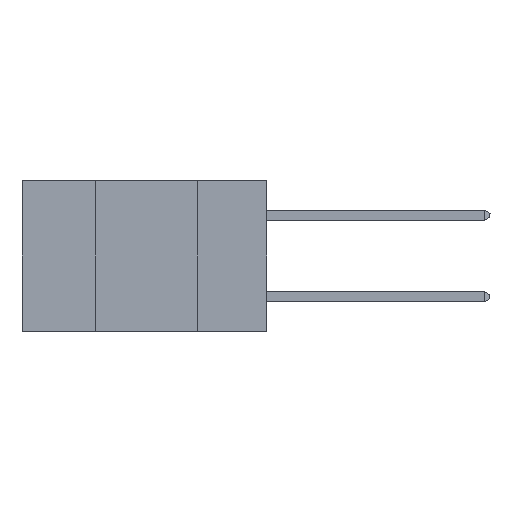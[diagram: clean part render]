
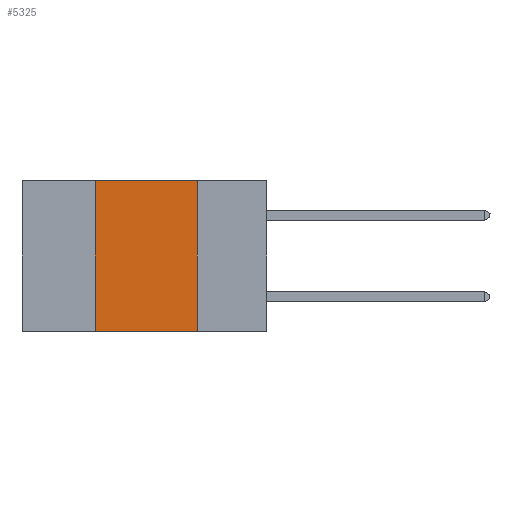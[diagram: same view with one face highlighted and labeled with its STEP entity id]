
A CAD part, left-side view. The second image highlights one B-rep face of the part: STEP entity #5325.
In plain terms, the highlighted planar face has unit normal (-1, 0, 0).
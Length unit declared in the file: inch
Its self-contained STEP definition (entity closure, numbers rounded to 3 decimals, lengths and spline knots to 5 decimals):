
#87 = DIRECTION ( 'NONE',  ( 0., -1., 0. ) ) ;
#696 = ORIENTED_EDGE ( 'NONE', *, *, #19331, .F. ) ;
#1381 = ORIENTED_EDGE ( 'NONE', *, *, #11304, .F. ) ;
#1955 = CARTESIAN_POINT ( 'NONE',  ( 0., 0.6, 0. ) ) ;
#4219 = CARTESIAN_POINT ( 'NONE',  ( 0., 0.17, -0.37 ) ) ;
#5291 = CARTESIAN_POINT ( 'NONE',  ( 0., 0.42, 0. ) ) ;
#5325 = ADVANCED_FACE ( 'NONE', ( #12590 ), #6819, .F. ) ;
#5712 = LINE ( 'NONE', #8011, #13206 ) ;
#6655 = DIRECTION ( 'NONE',  ( 0., 0., -1. ) ) ;
#6819 = PLANE ( 'NONE',  #17842 ) ;
#7284 = VERTEX_POINT ( 'NONE', #9125 ) ;
#7323 = DIRECTION ( 'NONE',  ( 1., 0., 0. ) ) ;
#7346 = VECTOR ( 'NONE', #11225, 39.37008 ) ;
#8011 = CARTESIAN_POINT ( 'NONE',  ( 0., 0.6, -0.37 ) ) ;
#8307 = DIRECTION ( 'NONE',  ( 0., 0., 1. ) ) ;
#8424 = ORIENTED_EDGE ( 'NONE', *, *, #16212, .F. ) ;
#8816 = VERTEX_POINT ( 'NONE', #12706 ) ;
#9031 = ORIENTED_EDGE ( 'NONE', *, *, #18347, .T. ) ;
#9125 = CARTESIAN_POINT ( 'NONE',  ( 0., 0.42, 0. ) ) ;
#10148 = DIRECTION ( 'NONE',  ( 0., 0., -1. ) ) ;
#10223 = VERTEX_POINT ( 'NONE', #4219 ) ;
#11225 = DIRECTION ( 'NONE',  ( 0., -1., 0. ) ) ;
#11304 = EDGE_CURVE ( 'NONE', #15109, #7284, #18231, .T. ) ;
#11358 = VECTOR ( 'NONE', #10148, 39.37008 ) ;
#12590 = FACE_OUTER_BOUND ( 'NONE', #13124, .T. ) ;
#12706 = CARTESIAN_POINT ( 'NONE',  ( 0., 0.17, 0. ) ) ;
#13124 = EDGE_LOOP ( 'NONE', ( #8424, #696, #1381, #9031 ) ) ;
#13206 = VECTOR ( 'NONE', #87, 39.37008 ) ;
#15109 = VERTEX_POINT ( 'NONE', #18492 ) ;
#16212 = EDGE_CURVE ( 'NONE', #8816, #10223, #19399, .T. ) ;
#17368 = CARTESIAN_POINT ( 'NONE',  ( 0., 0.17, 0. ) ) ;
#17842 = AXIS2_PLACEMENT_3D ( 'NONE', #18925, #7323, #6655 ) ;
#18231 = LINE ( 'NONE', #5291, #18676 ) ;
#18347 = EDGE_CURVE ( 'NONE', #15109, #10223, #5712, .T. ) ;
#18492 = CARTESIAN_POINT ( 'NONE',  ( 0., 0.42, -0.37 ) ) ;
#18676 = VECTOR ( 'NONE', #8307, 39.37008 ) ;
#18925 = CARTESIAN_POINT ( 'NONE',  ( 0., 0.6, 0. ) ) ;
#19331 = EDGE_CURVE ( 'NONE', #7284, #8816, #19407, .T. ) ;
#19399 = LINE ( 'NONE', #17368, #11358 ) ;
#19407 = LINE ( 'NONE', #1955, #7346 ) ;
